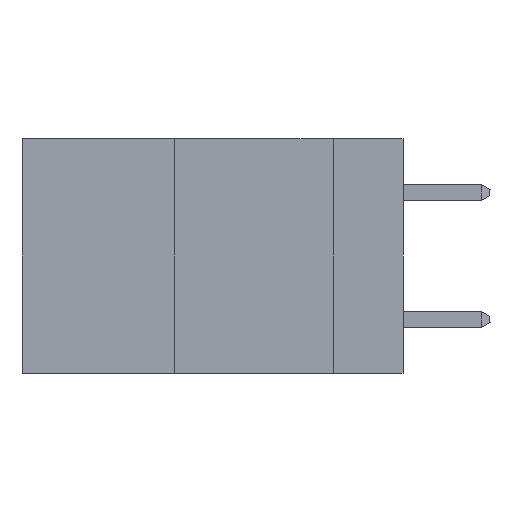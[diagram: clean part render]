
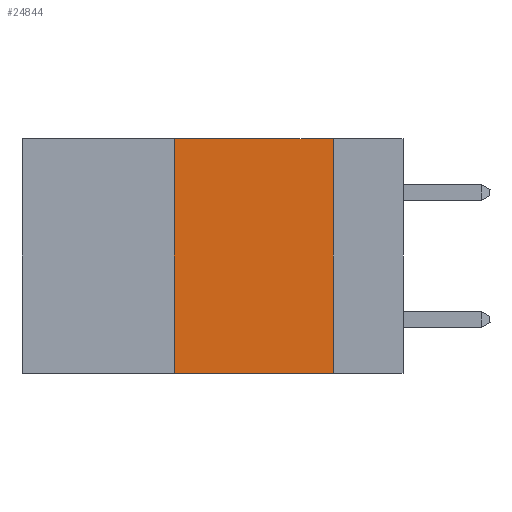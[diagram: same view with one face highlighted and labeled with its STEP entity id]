
A CAD part, left-side view. The second image highlights one B-rep face of the part: STEP entity #24844.
In plain terms, the highlighted planar face has unit normal (-1, 0, 0).
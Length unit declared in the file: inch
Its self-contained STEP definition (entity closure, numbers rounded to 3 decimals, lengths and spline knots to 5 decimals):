
#415 = AXIS2_PLACEMENT_3D ( 'NONE', #1315, #3881, #13739 ) ;
#1315 = CARTESIAN_POINT ( 'NONE',  ( 0., 0.6, 0. ) ) ;
#1766 = VECTOR ( 'NONE', #14248, 39.37008 ) ;
#1858 = VECTOR ( 'NONE', #14534, 39.37008 ) ;
#3779 = PLANE ( 'NONE',  #415 ) ;
#3881 = DIRECTION ( 'NONE',  ( 1., 0., 0. ) ) ;
#4165 = CARTESIAN_POINT ( 'NONE',  ( 0., 0.6, -0.37 ) ) ;
#4794 = ORIENTED_EDGE ( 'NONE', *, *, #29958, .F. ) ;
#6212 = DIRECTION ( 'NONE',  ( 0., 0., 1. ) ) ;
#7442 = ORIENTED_EDGE ( 'NONE', *, *, #12433, .F. ) ;
#8141 = LINE ( 'NONE', #4165, #1766 ) ;
#9224 = CARTESIAN_POINT ( 'NONE',  ( 0., 0.11, 0. ) ) ;
#10977 = CARTESIAN_POINT ( 'NONE',  ( 0., 0.36, 0. ) ) ;
#11695 = CARTESIAN_POINT ( 'NONE',  ( 0., 0.6, 0. ) ) ;
#12433 = EDGE_CURVE ( 'NONE', #15455, #17956, #25202, .T. ) ;
#13739 = DIRECTION ( 'NONE',  ( 0., 0., -1. ) ) ;
#14248 = DIRECTION ( 'NONE',  ( 0., -1., 0. ) ) ;
#14534 = DIRECTION ( 'NONE',  ( 0., -1., 0. ) ) ;
#14719 = DIRECTION ( 'NONE',  ( 0., 0., -1. ) ) ;
#15455 = VERTEX_POINT ( 'NONE', #26789 ) ;
#15989 = EDGE_CURVE ( 'NONE', #15455, #23790, #8141, .T. ) ;
#17956 = VERTEX_POINT ( 'NONE', #27166 ) ;
#18686 = LINE ( 'NONE', #11695, #1858 ) ;
#20833 = EDGE_LOOP ( 'NONE', ( #30910, #4794, #7442, #24039 ) ) ;
#21021 = FACE_OUTER_BOUND ( 'NONE', #20833, .T. ) ;
#23790 = VERTEX_POINT ( 'NONE', #25641 ) ;
#24039 = ORIENTED_EDGE ( 'NONE', *, *, #15989, .T. ) ;
#24844 = ADVANCED_FACE ( 'NONE', ( #21021 ), #3779, .F. ) ;
#25202 = LINE ( 'NONE', #10977, #30820 ) ;
#25641 = CARTESIAN_POINT ( 'NONE',  ( 0., 0.11, -0.37 ) ) ;
#25763 = LINE ( 'NONE', #9224, #28568 ) ;
#26789 = CARTESIAN_POINT ( 'NONE',  ( 0., 0.36, -0.37 ) ) ;
#27166 = CARTESIAN_POINT ( 'NONE',  ( 0., 0.36, 0. ) ) ;
#28568 = VECTOR ( 'NONE', #14719, 39.37008 ) ;
#29958 = EDGE_CURVE ( 'NONE', #17956, #32960, #18686, .T. ) ;
#30223 = CARTESIAN_POINT ( 'NONE',  ( 0., 0.11, 0. ) ) ;
#30621 = EDGE_CURVE ( 'NONE', #32960, #23790, #25763, .T. ) ;
#30820 = VECTOR ( 'NONE', #6212, 39.37008 ) ;
#30910 = ORIENTED_EDGE ( 'NONE', *, *, #30621, .F. ) ;
#32960 = VERTEX_POINT ( 'NONE', #30223 ) ;
